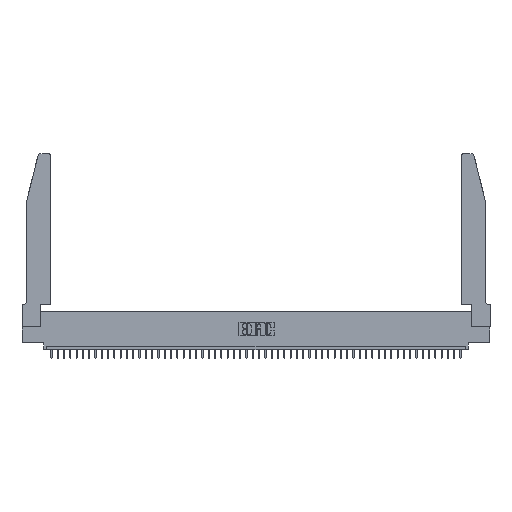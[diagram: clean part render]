
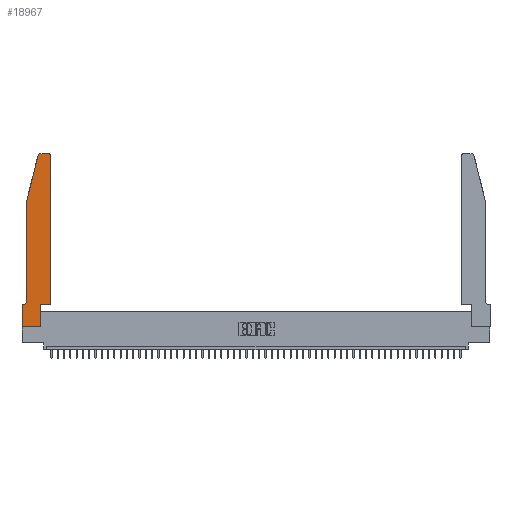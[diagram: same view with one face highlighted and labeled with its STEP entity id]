
A CAD part, top view. The second image highlights one B-rep face of the part: STEP entity #18967.
In plain terms, the highlighted planar face has unit normal (0, 0, 1).
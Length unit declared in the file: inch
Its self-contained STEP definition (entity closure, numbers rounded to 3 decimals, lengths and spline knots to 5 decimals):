
#882 = DIRECTION ( 'NONE',  ( 1., 0., 0. ) ) ;
#885 = EDGE_CURVE ( 'NONE', #43937, #21633, #7733, .T. ) ;
#891 = DIRECTION ( 'NONE',  ( 1., 0., 0. ) ) ;
#985 = VECTOR ( 'NONE', #8944, 39.37008 ) ;
#1088 = ORIENTED_EDGE ( 'NONE', *, *, #10413, .T. ) ;
#1092 = CIRCLE ( 'NONE', #37614, 0.07 ) ;
#1257 = VERTEX_POINT ( 'NONE', #43854 ) ;
#1904 = CIRCLE ( 'NONE', #5249, 0.03 ) ;
#2306 = VECTOR ( 'NONE', #36618, 39.37008 ) ;
#2357 = VERTEX_POINT ( 'NONE', #25206 ) ;
#3176 = ORIENTED_EDGE ( 'NONE', *, *, #6525, .T. ) ;
#3509 = CARTESIAN_POINT ( 'NONE',  ( 0., 0., 0.37 ) ) ;
#3675 = DIRECTION ( 'NONE',  ( 1., 0., 0. ) ) ;
#4148 = DIRECTION ( 'NONE',  ( -0.239, -0.971, 0. ) ) ;
#4267 = DIRECTION ( 'NONE',  ( 0., 1., 0. ) ) ;
#4317 = EDGE_CURVE ( 'NONE', #2357, #32775, #4791, .T. ) ;
#4791 = LINE ( 'NONE', #48756, #985 ) ;
#4803 = ORIENTED_EDGE ( 'NONE', *, *, #31092, .T. ) ;
#5249 = AXIS2_PLACEMENT_3D ( 'NONE', #7825, #23405, #3675 ) ;
#5294 = CARTESIAN_POINT ( 'NONE',  ( 0., 0., 0.37 ) ) ;
#5321 = CARTESIAN_POINT ( 'NONE',  ( 0.4205, 2.75, 0.37 ) ) ;
#6525 = EDGE_CURVE ( 'NONE', #32775, #43937, #1092, .T. ) ;
#6829 = EDGE_CURVE ( 'NONE', #30126, #35113, #1904, .T. ) ;
#7733 = LINE ( 'NONE', #32152, #46607 ) ;
#7825 = CARTESIAN_POINT ( 'NONE',  ( 0.4205, 2.72, 0.37 ) ) ;
#7860 = ORIENTED_EDGE ( 'NONE', *, *, #41461, .T. ) ;
#8919 = VERTEX_POINT ( 'NONE', #3509 ) ;
#8944 = DIRECTION ( 'NONE',  ( 0., -1., 0. ) ) ;
#9419 = CARTESIAN_POINT ( 'NONE',  ( 0., 0.35, 0.37 ) ) ;
#9555 = LINE ( 'NONE', #26199, #35523 ) ;
#10235 = ORIENTED_EDGE ( 'NONE', *, *, #43237, .T. ) ;
#10413 = EDGE_CURVE ( 'NONE', #8919, #36875, #48488, .T. ) ;
#10706 = CIRCLE ( 'NONE', #20694, 0.03 ) ;
#11163 = CARTESIAN_POINT ( 'NONE',  ( 0.4505, 2.72, 0.37 ) ) ;
#13143 = CARTESIAN_POINT ( 'NONE',  ( 0., 0., 0.37 ) ) ;
#16799 = CARTESIAN_POINT ( 'NONE',  ( 0.2865, 0., 0.37 ) ) ;
#16871 = EDGE_CURVE ( 'NONE', #21633, #8919, #36874, .T. ) ;
#16937 = DIRECTION ( 'NONE',  ( -1., 0., 0. ) ) ;
#17934 = VERTEX_POINT ( 'NONE', #22913 ) ;
#18794 = LINE ( 'NONE', #46141, #25632 ) ;
#18967 = ADVANCED_FACE ( 'NONE', ( #40675 ), #37507, .T. ) ;
#19967 = CARTESIAN_POINT ( 'NONE',  ( 0., 0.35, 0.37 ) ) ;
#20215 = EDGE_CURVE ( 'NONE', #35113, #1257, #18794, .T. ) ;
#20694 = AXIS2_PLACEMENT_3D ( 'NONE', #27685, #28191, #891 ) ;
#20862 = DIRECTION ( 'NONE',  ( 0., 0., 1. ) ) ;
#21633 = VERTEX_POINT ( 'NONE', #19967 ) ;
#21674 = VERTEX_POINT ( 'NONE', #38029 ) ;
#22076 = ORIENTED_EDGE ( 'NONE', *, *, #6829, .T. ) ;
#22441 = DIRECTION ( 'NONE',  ( -1., 0., 0. ) ) ;
#22913 = CARTESIAN_POINT ( 'NONE',  ( 0.4505, 0.35, 0.37 ) ) ;
#23393 = CARTESIAN_POINT ( 'NONE',  ( 0.0755, 0.42, 0.37 ) ) ;
#23405 = DIRECTION ( 'NONE',  ( 0., 0., 1. ) ) ;
#23567 = ORIENTED_EDGE ( 'NONE', *, *, #20215, .T. ) ;
#23636 = CARTESIAN_POINT ( 'NONE',  ( 0.0755, 2., 0.37 ) ) ;
#23649 = EDGE_LOOP ( 'NONE', ( #23567, #4803, #45967, #27632, #3176, #41518, #34024, #1088, #7860, #40973, #10235, #22076 ) ) ;
#25206 = CARTESIAN_POINT ( 'NONE',  ( 0.0755, 2., 0.37 ) ) ;
#25632 = VECTOR ( 'NONE', #22441, 39.37008 ) ;
#26199 = CARTESIAN_POINT ( 'NONE',  ( 0.4505, 0.35, 0.37 ) ) ;
#27632 = ORIENTED_EDGE ( 'NONE', *, *, #4317, .T. ) ;
#27685 = CARTESIAN_POINT ( 'NONE',  ( 0.284, 2.72, 0.37 ) ) ;
#28191 = DIRECTION ( 'NONE',  ( 0., 0., 1. ) ) ;
#29182 = EDGE_CURVE ( 'NONE', #33065, #17934, #9555, .T. ) ;
#30126 = VERTEX_POINT ( 'NONE', #11163 ) ;
#30397 = VECTOR ( 'NONE', #47509, 39.37008 ) ;
#31092 = EDGE_CURVE ( 'NONE', #1257, #21674, #10706, .T. ) ;
#31115 = CARTESIAN_POINT ( 'NONE',  ( 0.2865, 0.35, 0.37 ) ) ;
#31820 = LINE ( 'NONE', #34960, #42046 ) ;
#32152 = CARTESIAN_POINT ( 'NONE',  ( 0.0755, 0.35, 0.37 ) ) ;
#32775 = VERTEX_POINT ( 'NONE', #23393 ) ;
#33017 = AXIS2_PLACEMENT_3D ( 'NONE', #9419, #20862, #37006 ) ;
#33065 = VERTEX_POINT ( 'NONE', #37425 ) ;
#33819 = DIRECTION ( 'NONE',  ( 0., 0., -1. ) ) ;
#34024 = ORIENTED_EDGE ( 'NONE', *, *, #16871, .T. ) ;
#34960 = CARTESIAN_POINT ( 'NONE',  ( 0.4505, 0.35, 0.37 ) ) ;
#35113 = VERTEX_POINT ( 'NONE', #5321 ) ;
#35523 = VECTOR ( 'NONE', #49619, 39.37008 ) ;
#36618 = DIRECTION ( 'NONE',  ( 0., -1., 0. ) ) ;
#36874 = LINE ( 'NONE', #13143, #2306 ) ;
#36875 = VERTEX_POINT ( 'NONE', #16799 ) ;
#37006 = DIRECTION ( 'NONE',  ( 1., 0., 0. ) ) ;
#37425 = CARTESIAN_POINT ( 'NONE',  ( 0.2865, 0.35, 0.37 ) ) ;
#37499 = CARTESIAN_POINT ( 'NONE',  ( 0.0055, 0.42, 0.37 ) ) ;
#37507 = PLANE ( 'NONE',  #33017 ) ;
#37614 = AXIS2_PLACEMENT_3D ( 'NONE', #37499, #33819, #16937 ) ;
#37984 = CARTESIAN_POINT ( 'NONE',  ( 0.0055, 0.35, 0.37 ) ) ;
#38029 = CARTESIAN_POINT ( 'NONE',  ( 0.25487, 2.72718, 0.37 ) ) ;
#39796 = LINE ( 'NONE', #23636, #40624 ) ;
#40287 = VECTOR ( 'NONE', #882, 39.37008 ) ;
#40624 = VECTOR ( 'NONE', #4148, 39.37008 ) ;
#40675 = FACE_OUTER_BOUND ( 'NONE', #23649, .T. ) ;
#40973 = ORIENTED_EDGE ( 'NONE', *, *, #29182, .T. ) ;
#41461 = EDGE_CURVE ( 'NONE', #36875, #33065, #51404, .T. ) ;
#41518 = ORIENTED_EDGE ( 'NONE', *, *, #885, .T. ) ;
#42046 = VECTOR ( 'NONE', #4267, 39.37008 ) ;
#43237 = EDGE_CURVE ( 'NONE', #17934, #30126, #31820, .T. ) ;
#43854 = CARTESIAN_POINT ( 'NONE',  ( 0.284, 2.75, 0.37 ) ) ;
#43937 = VERTEX_POINT ( 'NONE', #37984 ) ;
#45967 = ORIENTED_EDGE ( 'NONE', *, *, #46955, .T. ) ;
#46141 = CARTESIAN_POINT ( 'NONE',  ( 0.2605, 2.75, 0.37 ) ) ;
#46607 = VECTOR ( 'NONE', #49362, 39.37008 ) ;
#46955 = EDGE_CURVE ( 'NONE', #21674, #2357, #39796, .T. ) ;
#47509 = DIRECTION ( 'NONE',  ( 0., 1., 0. ) ) ;
#48488 = LINE ( 'NONE', #5294, #40287 ) ;
#48756 = CARTESIAN_POINT ( 'NONE',  ( 0.0755, 2., 0.37 ) ) ;
#49362 = DIRECTION ( 'NONE',  ( -1., 0., 0. ) ) ;
#49619 = DIRECTION ( 'NONE',  ( 1., 0., 0. ) ) ;
#51404 = LINE ( 'NONE', #31115, #30397 ) ;
